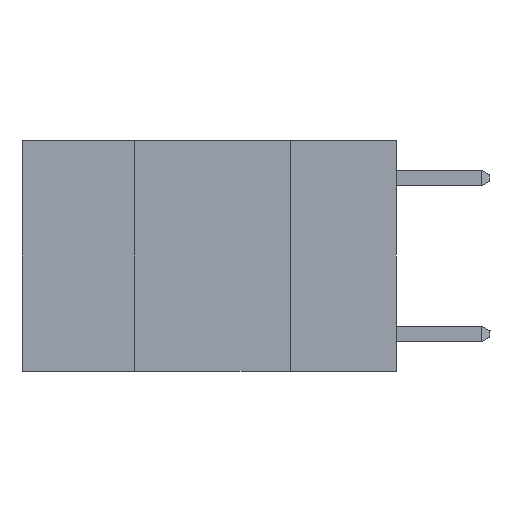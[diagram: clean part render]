
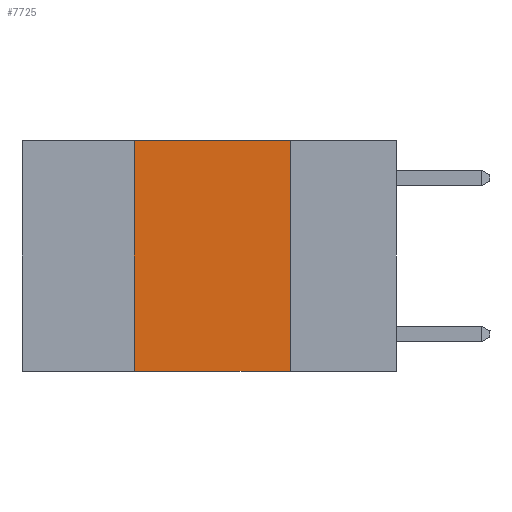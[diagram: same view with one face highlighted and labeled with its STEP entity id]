
A CAD part, left-side view. The second image highlights one B-rep face of the part: STEP entity #7725.
In plain terms, the highlighted planar face has unit normal (-1, 0, 0).
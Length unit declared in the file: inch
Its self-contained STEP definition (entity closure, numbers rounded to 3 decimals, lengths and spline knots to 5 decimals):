
#190 = EDGE_CURVE ( 'NONE', #766, #3384, #5762, .T. ) ;
#766 = VERTEX_POINT ( 'NONE', #8097 ) ;
#1058 = AXIS2_PLACEMENT_3D ( 'NONE', #2930, #8292, #3667 ) ;
#1060 = EDGE_CURVE ( 'NONE', #766, #8695, #7505, .T. ) ;
#1406 = ORIENTED_EDGE ( 'NONE', *, *, #1060, .T. ) ;
#1423 = DIRECTION ( 'NONE',  ( 0., -1., 0. ) ) ;
#1598 = CARTESIAN_POINT ( 'NONE',  ( 0., 0.42, 0. ) ) ;
#1679 = ORIENTED_EDGE ( 'NONE', *, *, #8775, .F. ) ;
#1818 = EDGE_CURVE ( 'NONE', #3384, #9601, #6170, .T. ) ;
#2928 = CARTESIAN_POINT ( 'NONE',  ( 0., 0.42, 0. ) ) ;
#2930 = CARTESIAN_POINT ( 'NONE',  ( 0., 0.6, 0. ) ) ;
#3309 = CARTESIAN_POINT ( 'NONE',  ( 0., 0.6, -0.37 ) ) ;
#3347 = CARTESIAN_POINT ( 'NONE',  ( 0., 0.17, -0.37 ) ) ;
#3384 = VERTEX_POINT ( 'NONE', #2928 ) ;
#3406 = VECTOR ( 'NONE', #1423, 39.37008 ) ;
#3667 = DIRECTION ( 'NONE',  ( 0., 0., -1. ) ) ;
#4199 = CARTESIAN_POINT ( 'NONE',  ( 0., 0.17, 0. ) ) ;
#4918 = DIRECTION ( 'NONE',  ( 0., 0., 1. ) ) ;
#4926 = DIRECTION ( 'NONE',  ( 0., 0., -1. ) ) ;
#5303 = ORIENTED_EDGE ( 'NONE', *, *, #190, .F. ) ;
#5762 = LINE ( 'NONE', #1598, #9665 ) ;
#5879 = FACE_OUTER_BOUND ( 'NONE', #8761, .T. ) ;
#6170 = LINE ( 'NONE', #7097, #7876 ) ;
#6177 = VECTOR ( 'NONE', #4926, 39.37008 ) ;
#7097 = CARTESIAN_POINT ( 'NONE',  ( 0., 0.6, 0. ) ) ;
#7505 = LINE ( 'NONE', #3309, #3406 ) ;
#7506 = PLANE ( 'NONE',  #1058 ) ;
#7681 = DIRECTION ( 'NONE',  ( 0., -1., 0. ) ) ;
#7725 = ADVANCED_FACE ( 'NONE', ( #5879 ), #7506, .F. ) ;
#7876 = VECTOR ( 'NONE', #7681, 39.37008 ) ;
#8047 = CARTESIAN_POINT ( 'NONE',  ( 0., 0.17, 0. ) ) ;
#8097 = CARTESIAN_POINT ( 'NONE',  ( 0., 0.42, -0.37 ) ) ;
#8292 = DIRECTION ( 'NONE',  ( 1., 0., 0. ) ) ;
#8354 = LINE ( 'NONE', #8047, #6177 ) ;
#8695 = VERTEX_POINT ( 'NONE', #3347 ) ;
#8761 = EDGE_LOOP ( 'NONE', ( #1679, #9798, #5303, #1406 ) ) ;
#8775 = EDGE_CURVE ( 'NONE', #9601, #8695, #8354, .T. ) ;
#9601 = VERTEX_POINT ( 'NONE', #4199 ) ;
#9665 = VECTOR ( 'NONE', #4918, 39.37008 ) ;
#9798 = ORIENTED_EDGE ( 'NONE', *, *, #1818, .F. ) ;
